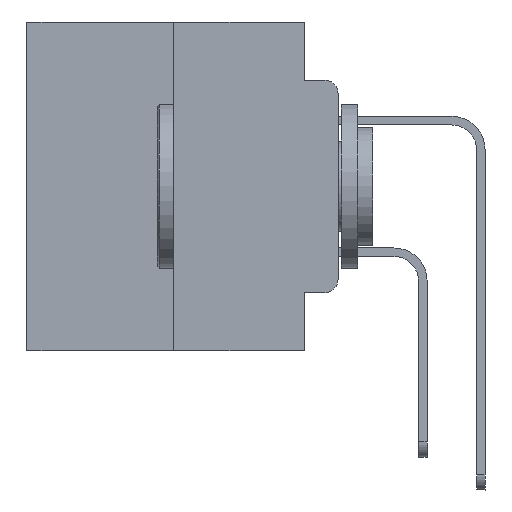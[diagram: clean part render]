
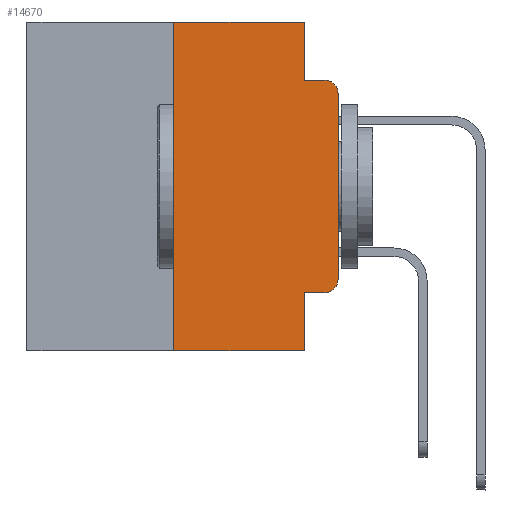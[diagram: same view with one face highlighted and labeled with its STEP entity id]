
A CAD part, left-side view. The second image highlights one B-rep face of the part: STEP entity #14670.
In plain terms, the highlighted planar face has unit normal (-1, 0, 0).
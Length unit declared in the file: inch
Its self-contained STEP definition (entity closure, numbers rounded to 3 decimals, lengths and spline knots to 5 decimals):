
#140 = LINE ( 'NONE', #2047, #13656 ) ;
#322 = DIRECTION ( 'NONE',  ( 0., 0., -1. ) ) ;
#829 = EDGE_CURVE ( 'NONE', #17892, #20343, #17082, .T. ) ;
#1567 = CARTESIAN_POINT ( 'NONE',  ( 0., 0.25, 0. ) ) ;
#2024 = CARTESIAN_POINT ( 'NONE',  ( 0., 0.051, -0.0885 ) ) ;
#2047 = CARTESIAN_POINT ( 'NONE',  ( 0., 0.051, 0. ) ) ;
#2104 = ORIENTED_EDGE ( 'NONE', *, *, #6291, .T. ) ;
#2162 = AXIS2_PLACEMENT_3D ( 'NONE', #5761, #25526, #10345 ) ;
#2924 = ORIENTED_EDGE ( 'NONE', *, *, #9148, .T. ) ;
#3203 = VERTEX_POINT ( 'NONE', #22891 ) ;
#3501 = VECTOR ( 'NONE', #8090, 39.37008 ) ;
#4608 = ORIENTED_EDGE ( 'NONE', *, *, #10714, .T. ) ;
#4609 = FACE_OUTER_BOUND ( 'NONE', #7980, .T. ) ;
#4899 = CARTESIAN_POINT ( 'NONE',  ( 0., 0., -0.3915 ) ) ;
#5123 = VERTEX_POINT ( 'NONE', #4899 ) ;
#5761 = CARTESIAN_POINT ( 'NONE',  ( 0., 0.02, -0.1085 ) ) ;
#6168 = DIRECTION ( 'NONE',  ( 0., -1., 0. ) ) ;
#6181 = CARTESIAN_POINT ( 'NONE',  ( 0., 0.02, -0.0885 ) ) ;
#6226 = DIRECTION ( 'NONE',  ( 0., -1., 0. ) ) ;
#6282 = CARTESIAN_POINT ( 'NONE',  ( 0., 0.051, -0.4115 ) ) ;
#6291 = EDGE_CURVE ( 'NONE', #10686, #3203, #17482, .T. ) ;
#7104 = CARTESIAN_POINT ( 'NONE',  ( 0., 0., 0. ) ) ;
#7268 = EDGE_CURVE ( 'NONE', #10686, #17892, #17271, .T. ) ;
#7599 = VECTOR ( 'NONE', #9751, 39.37008 ) ;
#7607 = CARTESIAN_POINT ( 'NONE',  ( 0., 0., -0.1085 ) ) ;
#7980 = EDGE_LOOP ( 'NONE', ( #8834, #4608, #27988, #16913, #8558, #28794, #2104, #10716, #2924, #23139 ) ) ;
#8090 = DIRECTION ( 'NONE',  ( 0., 0., 1. ) ) ;
#8440 = EDGE_CURVE ( 'NONE', #20018, #5123, #21181, .T. ) ;
#8558 = ORIENTED_EDGE ( 'NONE', *, *, #829, .F. ) ;
#8834 = ORIENTED_EDGE ( 'NONE', *, *, #18847, .T. ) ;
#8898 = PLANE ( 'NONE',  #23976 ) ;
#9148 = EDGE_CURVE ( 'NONE', #21751, #20018, #15692, .T. ) ;
#9751 = DIRECTION ( 'NONE',  ( 0., 0., 1. ) ) ;
#10306 = VECTOR ( 'NONE', #19257, 39.37008 ) ;
#10345 = DIRECTION ( 'NONE',  ( 0., 0., -1. ) ) ;
#10686 = VERTEX_POINT ( 'NONE', #21405 ) ;
#10714 = EDGE_CURVE ( 'NONE', #25190, #10837, #20092, .T. ) ;
#10716 = ORIENTED_EDGE ( 'NONE', *, *, #15182, .F. ) ;
#10837 = VERTEX_POINT ( 'NONE', #6181 ) ;
#11071 = LINE ( 'NONE', #2024, #19141 ) ;
#11130 = DIRECTION ( 'NONE',  ( 1., 0., 0. ) ) ;
#11171 = VECTOR ( 'NONE', #19819, 39.37008 ) ;
#12459 = LINE ( 'NONE', #25428, #10306 ) ;
#13656 = VECTOR ( 'NONE', #24781, 39.37008 ) ;
#14486 = EDGE_CURVE ( 'NONE', #20343, #21499, #12459, .T. ) ;
#14670 = ADVANCED_FACE ( 'NONE', ( #4609 ), #8898, .F. ) ;
#14759 = DIRECTION ( 'NONE',  ( 0., 0., -1. ) ) ;
#15182 = EDGE_CURVE ( 'NONE', #21751, #3203, #140, .T. ) ;
#15692 = LINE ( 'NONE', #22012, #11171 ) ;
#16115 = VECTOR ( 'NONE', #6226, 39.37008 ) ;
#16913 = ORIENTED_EDGE ( 'NONE', *, *, #14486, .F. ) ;
#17082 = LINE ( 'NONE', #28701, #22059 ) ;
#17129 = DIRECTION ( 'NONE',  ( -1., 0., 0. ) ) ;
#17271 = LINE ( 'NONE', #1567, #3501 ) ;
#17482 = LINE ( 'NONE', #26582, #16115 ) ;
#17892 = VERTEX_POINT ( 'NONE', #26679 ) ;
#17929 = CARTESIAN_POINT ( 'NONE',  ( 0., 0.473, 0. ) ) ;
#18354 = LINE ( 'NONE', #7104, #7599 ) ;
#18847 = EDGE_CURVE ( 'NONE', #5123, #25190, #18354, .T. ) ;
#19141 = VECTOR ( 'NONE', #6168, 39.37008 ) ;
#19257 = DIRECTION ( 'NONE',  ( 0., 0., -1. ) ) ;
#19819 = DIRECTION ( 'NONE',  ( 0., -1., 0. ) ) ;
#20018 = VERTEX_POINT ( 'NONE', #23257 ) ;
#20092 = CIRCLE ( 'NONE', #2162, 0.02 ) ;
#20343 = VERTEX_POINT ( 'NONE', #20440 ) ;
#20440 = CARTESIAN_POINT ( 'NONE',  ( 0., 0.051, 0. ) ) ;
#21181 = CIRCLE ( 'NONE', #26831, 0.02 ) ;
#21405 = CARTESIAN_POINT ( 'NONE',  ( 0., 0.25, -0.5 ) ) ;
#21499 = VERTEX_POINT ( 'NONE', #26860 ) ;
#21671 = CARTESIAN_POINT ( 'NONE',  ( 0., 0.02, -0.3915 ) ) ;
#21751 = VERTEX_POINT ( 'NONE', #6282 ) ;
#22012 = CARTESIAN_POINT ( 'NONE',  ( 0., 0.051, -0.4115 ) ) ;
#22059 = VECTOR ( 'NONE', #28844, 39.37008 ) ;
#22891 = CARTESIAN_POINT ( 'NONE',  ( 0., 0.051, -0.5 ) ) ;
#23139 = ORIENTED_EDGE ( 'NONE', *, *, #8440, .T. ) ;
#23257 = CARTESIAN_POINT ( 'NONE',  ( 0., 0.02, -0.4115 ) ) ;
#23976 = AXIS2_PLACEMENT_3D ( 'NONE', #17929, #11130, #322 ) ;
#24781 = DIRECTION ( 'NONE',  ( 0., 0., -1. ) ) ;
#25190 = VERTEX_POINT ( 'NONE', #7607 ) ;
#25428 = CARTESIAN_POINT ( 'NONE',  ( 0., 0.051, 0. ) ) ;
#25526 = DIRECTION ( 'NONE',  ( -1., 0., 0. ) ) ;
#26582 = CARTESIAN_POINT ( 'NONE',  ( 0., 0.473, -0.5 ) ) ;
#26679 = CARTESIAN_POINT ( 'NONE',  ( 0., 0.25, 0. ) ) ;
#26831 = AXIS2_PLACEMENT_3D ( 'NONE', #21671, #17129, #14759 ) ;
#26860 = CARTESIAN_POINT ( 'NONE',  ( 0., 0.051, -0.0885 ) ) ;
#27988 = ORIENTED_EDGE ( 'NONE', *, *, #28372, .F. ) ;
#28372 = EDGE_CURVE ( 'NONE', #21499, #10837, #11071, .T. ) ;
#28701 = CARTESIAN_POINT ( 'NONE',  ( 0., 0.473, 0. ) ) ;
#28794 = ORIENTED_EDGE ( 'NONE', *, *, #7268, .F. ) ;
#28844 = DIRECTION ( 'NONE',  ( 0., -1., 0. ) ) ;
